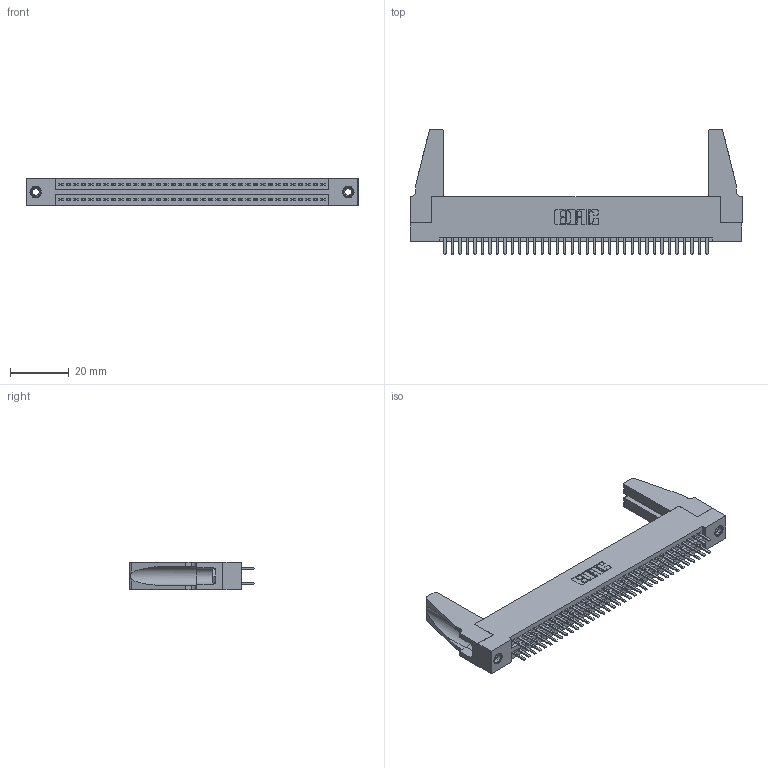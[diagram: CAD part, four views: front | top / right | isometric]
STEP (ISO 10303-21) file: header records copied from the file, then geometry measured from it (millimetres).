
FILE_DESCRIPTION (( 'STEP AP203' ), '1' );
FILE_NAME ('395-072-520-288.STEP', '2019-10-24T11:33:24', ( '' ), ( '' ), 'SwSTEP 2.0', 'SolidWorks 2016', '' );
FILE_SCHEMA (( 'CONFIG_CONTROL_DESIGN' ));
Length unit declared in the file: inch
Products named in the file (5): 345 Part_Flush Mounting Lugs - 0.156 Dia-TH; 345-292-001_345-293-120; 345-250-001_345-250-001-102; 345-220-078_345-220-088; 395-072-520-288
Assembly tree (77 placements, depth 2):
  395-072-520-288
    345 Part_Flush Mounting Lugs - 0.156 Dia-TH
    345-292-001_345-293-120  x72
    345-250-001_345-250-001-102  x2
    345-220-078_345-220-088  x2
Bounding box: 112.67 x 42.55 x 9.4 mm (x, y, z)
Volume: 14110.4 mm3; surface area: 18988.5 mm2
Topology: 77 solids, 77 shells, 4138 faces, 11959 edges, 7770 vertices
Faces by surface type: plane 2672, cylinder 1450, cone 12, torus 4
Entity records: 31316 total; most frequent: CARTESIAN_POINT 5262, ORIENTED_EDGE 5144, DIRECTION 4640, EDGE_CURVE 2572, VECTOR 2250, LINE 2250, VERTEX_POINT 1706, AXIS2_PLACEMENT_3D 1195
